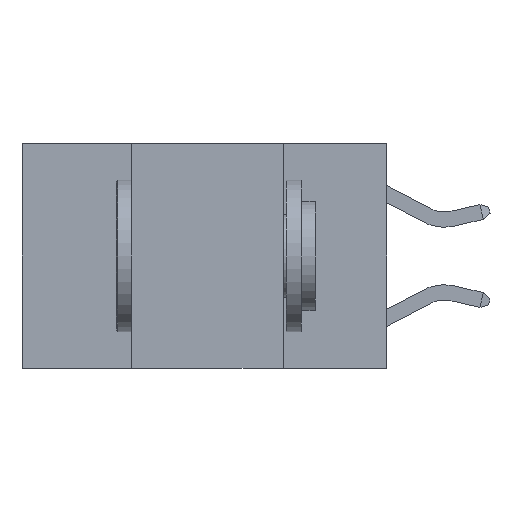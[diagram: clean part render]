
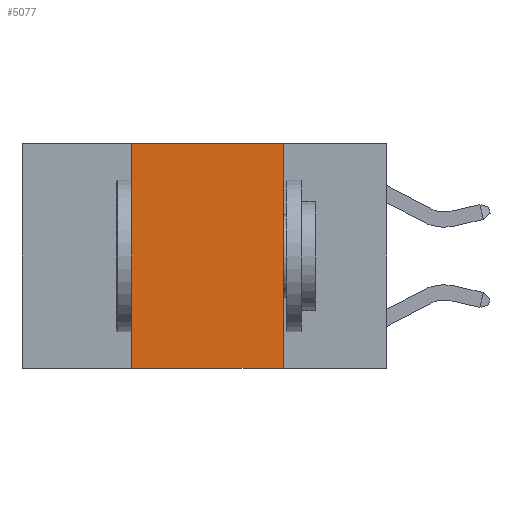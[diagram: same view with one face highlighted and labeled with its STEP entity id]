
A CAD part, left-side view. The second image highlights one B-rep face of the part: STEP entity #5077.
In plain terms, the highlighted planar face has unit normal (-1, 0, 0).
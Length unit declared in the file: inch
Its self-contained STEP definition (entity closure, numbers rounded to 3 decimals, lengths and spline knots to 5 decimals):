
#1180 = FACE_OUTER_BOUND ( 'NONE', #5407, .T. ) ;
#1503 = EDGE_CURVE ( 'NONE', #6023, #3001, #7762, .T. ) ;
#1577 = VECTOR ( 'NONE', #9807, 39.37008 ) ;
#1654 = CARTESIAN_POINT ( 'NONE',  ( 0., 0.17, 0. ) ) ;
#1878 = CARTESIAN_POINT ( 'NONE',  ( 0., 0.42, -0.37 ) ) ;
#2289 = VERTEX_POINT ( 'NONE', #3745 ) ;
#2476 = VECTOR ( 'NONE', #2979, 39.37008 ) ;
#2595 = ORIENTED_EDGE ( 'NONE', *, *, #2747, .T. ) ;
#2747 = EDGE_CURVE ( 'NONE', #5011, #2289, #8957, .T. ) ;
#2869 = DIRECTION ( 'NONE',  ( 0., 0., -1. ) ) ;
#2936 = EDGE_CURVE ( 'NONE', #5011, #6023, #9329, .T. ) ;
#2938 = CARTESIAN_POINT ( 'NONE',  ( 0., 0.6, -0.37 ) ) ;
#2979 = DIRECTION ( 'NONE',  ( 0., -1., 0. ) ) ;
#3001 = VERTEX_POINT ( 'NONE', #10462 ) ;
#3745 = CARTESIAN_POINT ( 'NONE',  ( 0., 0.17, -0.37 ) ) ;
#3857 = LINE ( 'NONE', #1654, #1577 ) ;
#3884 = CARTESIAN_POINT ( 'NONE',  ( 0., 0.42, 0. ) ) ;
#4776 = DIRECTION ( 'NONE',  ( 0., 0., 1. ) ) ;
#5011 = VERTEX_POINT ( 'NONE', #1878 ) ;
#5061 = ORIENTED_EDGE ( 'NONE', *, *, #10028, .F. ) ;
#5077 = ADVANCED_FACE ( 'NONE', ( #1180 ), #5334, .F. ) ;
#5087 = DIRECTION ( 'NONE',  ( 0., -1., 0. ) ) ;
#5175 = CARTESIAN_POINT ( 'NONE',  ( 0., 0.6, 0. ) ) ;
#5334 = PLANE ( 'NONE',  #10557 ) ;
#5407 = EDGE_LOOP ( 'NONE', ( #5061, #9076, #6986, #2595 ) ) ;
#5620 = VECTOR ( 'NONE', #5087, 39.37008 ) ;
#6023 = VERTEX_POINT ( 'NONE', #7299 ) ;
#6986 = ORIENTED_EDGE ( 'NONE', *, *, #2936, .F. ) ;
#7248 = VECTOR ( 'NONE', #4776, 39.37008 ) ;
#7299 = CARTESIAN_POINT ( 'NONE',  ( 0., 0.42, 0. ) ) ;
#7762 = LINE ( 'NONE', #5175, #5620 ) ;
#7763 = DIRECTION ( 'NONE',  ( 1., 0., 0. ) ) ;
#8957 = LINE ( 'NONE', #2938, #2476 ) ;
#9076 = ORIENTED_EDGE ( 'NONE', *, *, #1503, .F. ) ;
#9305 = CARTESIAN_POINT ( 'NONE',  ( 0., 0.6, 0. ) ) ;
#9329 = LINE ( 'NONE', #3884, #7248 ) ;
#9807 = DIRECTION ( 'NONE',  ( 0., 0., -1. ) ) ;
#10028 = EDGE_CURVE ( 'NONE', #3001, #2289, #3857, .T. ) ;
#10462 = CARTESIAN_POINT ( 'NONE',  ( 0., 0.17, 0. ) ) ;
#10557 = AXIS2_PLACEMENT_3D ( 'NONE', #9305, #7763, #2869 ) ;
